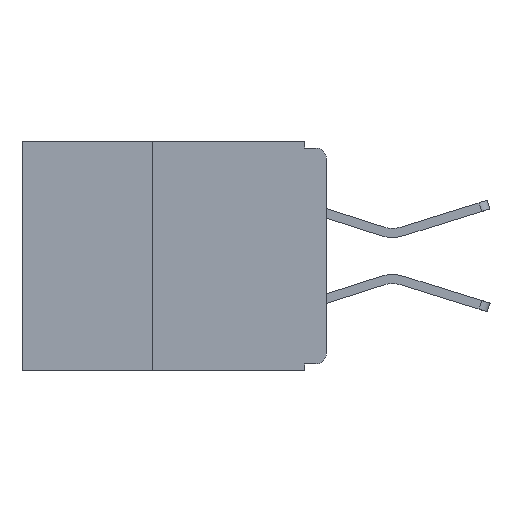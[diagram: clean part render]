
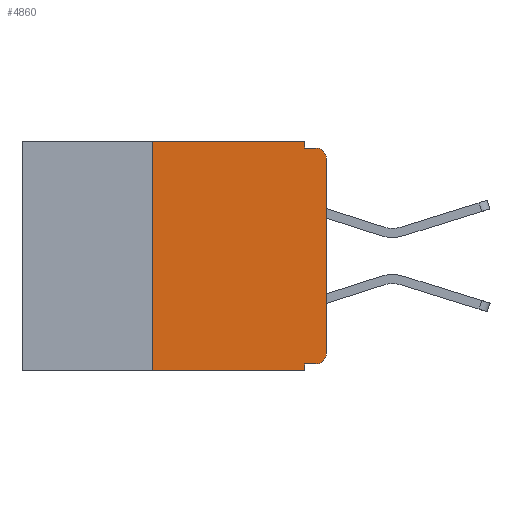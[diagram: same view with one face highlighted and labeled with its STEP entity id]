
A CAD part, left-side view. The second image highlights one B-rep face of the part: STEP entity #4860.
In plain terms, the highlighted planar face has unit normal (-1, 0, 0).
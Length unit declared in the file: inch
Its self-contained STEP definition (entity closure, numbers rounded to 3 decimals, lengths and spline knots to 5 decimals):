
#43 = LINE ( 'NONE', #23485, #11385 ) ;
#1338 = VERTEX_POINT ( 'NONE', #29481 ) ;
#1830 = LINE ( 'NONE', #26100, #28322 ) ;
#1840 = FACE_OUTER_BOUND ( 'NONE', #27056, .T. ) ;
#1933 = AXIS2_PLACEMENT_3D ( 'NONE', #18359, #2943, #20865 ) ;
#2165 = VERTEX_POINT ( 'NONE', #4716 ) ;
#2302 = VECTOR ( 'NONE', #6045, 39.37008 ) ;
#2535 = CARTESIAN_POINT ( 'NONE',  ( 0., 0.25, -0.33 ) ) ;
#2649 = CARTESIAN_POINT ( 'NONE',  ( 0., 0.25, -0.33 ) ) ;
#2943 = DIRECTION ( 'NONE',  ( -1., 0., 0. ) ) ;
#3326 = DIRECTION ( 'NONE',  ( 0., -1., 0. ) ) ;
#3347 = ORIENTED_EDGE ( 'NONE', *, *, #19460, .T. ) ;
#3734 = CARTESIAN_POINT ( 'NONE',  ( 0., 0.015, -0.025 ) ) ;
#4126 = VECTOR ( 'NONE', #15918, 39.37008 ) ;
#4716 = CARTESIAN_POINT ( 'NONE',  ( 0., 0., -0.305 ) ) ;
#4750 = CARTESIAN_POINT ( 'NONE',  ( 0., 0., -0.025 ) ) ;
#4860 = ADVANCED_FACE ( 'NONE', ( #1840 ), #25581, .F. ) ;
#4918 = EDGE_CURVE ( 'NONE', #14846, #13482, #27250, .T. ) ;
#5679 = ORIENTED_EDGE ( 'NONE', *, *, #11843, .F. ) ;
#6036 = VERTEX_POINT ( 'NONE', #6167 ) ;
#6045 = DIRECTION ( 'NONE',  ( 0., 0., -1. ) ) ;
#6167 = CARTESIAN_POINT ( 'NONE',  ( 0., 0.031, 0. ) ) ;
#6337 = DIRECTION ( 'NONE',  ( 0., 0., -1. ) ) ;
#6583 = EDGE_CURVE ( 'NONE', #7610, #16724, #1830, .T. ) ;
#6735 = ORIENTED_EDGE ( 'NONE', *, *, #13038, .F. ) ;
#7159 = VECTOR ( 'NONE', #10662, 39.37008 ) ;
#7420 = VERTEX_POINT ( 'NONE', #24932 ) ;
#7610 = VERTEX_POINT ( 'NONE', #21258 ) ;
#7653 = VECTOR ( 'NONE', #10467, 39.37008 ) ;
#9402 = CIRCLE ( 'NONE', #15820, 0.015 ) ;
#9878 = CARTESIAN_POINT ( 'NONE',  ( 0., 0.031, -0.33 ) ) ;
#10213 = LINE ( 'NONE', #18460, #4126 ) ;
#10467 = DIRECTION ( 'NONE',  ( 0., 0., 1. ) ) ;
#10662 = DIRECTION ( 'NONE',  ( 0., 1., 0. ) ) ;
#10884 = ORIENTED_EDGE ( 'NONE', *, *, #26653, .T. ) ;
#11244 = CARTESIAN_POINT ( 'NONE',  ( 0., 0.015, -0.01 ) ) ;
#11385 = VECTOR ( 'NONE', #28417, 39.37008 ) ;
#11645 = LINE ( 'NONE', #18712, #30720 ) ;
#11775 = CIRCLE ( 'NONE', #1933, 0.015 ) ;
#11843 = EDGE_CURVE ( 'NONE', #14846, #12485, #14467, .T. ) ;
#12485 = VERTEX_POINT ( 'NONE', #30921 ) ;
#13038 = EDGE_CURVE ( 'NONE', #1338, #7420, #13977, .T. ) ;
#13207 = ORIENTED_EDGE ( 'NONE', *, *, #20658, .F. ) ;
#13482 = VERTEX_POINT ( 'NONE', #9878 ) ;
#13977 = LINE ( 'NONE', #25725, #7159 ) ;
#14467 = LINE ( 'NONE', #2649, #7653 ) ;
#14846 = VERTEX_POINT ( 'NONE', #2535 ) ;
#15820 = AXIS2_PLACEMENT_3D ( 'NONE', #3734, #21602, #6337 ) ;
#15918 = DIRECTION ( 'NONE',  ( 0., 0., 1. ) ) ;
#16036 = AXIS2_PLACEMENT_3D ( 'NONE', #25434, #25361, #25319 ) ;
#16724 = VERTEX_POINT ( 'NONE', #11244 ) ;
#18359 = CARTESIAN_POINT ( 'NONE',  ( 0., 0.015, -0.305 ) ) ;
#18460 = CARTESIAN_POINT ( 'NONE',  ( 0., 0., 0. ) ) ;
#18712 = CARTESIAN_POINT ( 'NONE',  ( 0., 0.437, 0. ) ) ;
#18724 = EDGE_CURVE ( 'NONE', #6036, #7610, #43, .T. ) ;
#19101 = VERTEX_POINT ( 'NONE', #4750 ) ;
#19460 = EDGE_CURVE ( 'NONE', #19101, #16724, #9402, .T. ) ;
#20658 = EDGE_CURVE ( 'NONE', #12485, #6036, #11645, .T. ) ;
#20865 = DIRECTION ( 'NONE',  ( 0., 0., -1. ) ) ;
#21258 = CARTESIAN_POINT ( 'NONE',  ( 0., 0.031, -0.01 ) ) ;
#21354 = CARTESIAN_POINT ( 'NONE',  ( 0., 0.031, -0.33 ) ) ;
#21386 = ORIENTED_EDGE ( 'NONE', *, *, #4918, .T. ) ;
#21602 = DIRECTION ( 'NONE',  ( -1., 0., 0. ) ) ;
#23485 = CARTESIAN_POINT ( 'NONE',  ( 0., 0.031, 0. ) ) ;
#24553 = CARTESIAN_POINT ( 'NONE',  ( 0., 0.437, -0.33 ) ) ;
#24576 = DIRECTION ( 'NONE',  ( 0., -1., 0. ) ) ;
#24932 = CARTESIAN_POINT ( 'NONE',  ( 0., 0.031, -0.32 ) ) ;
#25319 = DIRECTION ( 'NONE',  ( 0., 0., -1. ) ) ;
#25361 = DIRECTION ( 'NONE',  ( 1., 0., 0. ) ) ;
#25434 = CARTESIAN_POINT ( 'NONE',  ( 0., 0.437, 0. ) ) ;
#25581 = PLANE ( 'NONE',  #16036 ) ;
#25725 = CARTESIAN_POINT ( 'NONE',  ( 0., 0., -0.32 ) ) ;
#25998 = DIRECTION ( 'NONE',  ( 0., -1., 0. ) ) ;
#26100 = CARTESIAN_POINT ( 'NONE',  ( 0., 0., -0.01 ) ) ;
#26457 = VECTOR ( 'NONE', #24576, 39.37008 ) ;
#26653 = EDGE_CURVE ( 'NONE', #1338, #2165, #11775, .T. ) ;
#26699 = EDGE_CURVE ( 'NONE', #2165, #19101, #10213, .T. ) ;
#26879 = ORIENTED_EDGE ( 'NONE', *, *, #30800, .F. ) ;
#27056 = EDGE_LOOP ( 'NONE', ( #27460, #3347, #27448, #29534, #13207, #5679, #21386, #26879, #6735, #10884 ) ) ;
#27250 = LINE ( 'NONE', #24553, #26457 ) ;
#27448 = ORIENTED_EDGE ( 'NONE', *, *, #6583, .F. ) ;
#27460 = ORIENTED_EDGE ( 'NONE', *, *, #26699, .T. ) ;
#28322 = VECTOR ( 'NONE', #25998, 39.37008 ) ;
#28416 = LINE ( 'NONE', #21354, #2302 ) ;
#28417 = DIRECTION ( 'NONE',  ( 0., 0., -1. ) ) ;
#29481 = CARTESIAN_POINT ( 'NONE',  ( 0., 0.015, -0.32 ) ) ;
#29534 = ORIENTED_EDGE ( 'NONE', *, *, #18724, .F. ) ;
#30720 = VECTOR ( 'NONE', #3326, 39.37008 ) ;
#30800 = EDGE_CURVE ( 'NONE', #7420, #13482, #28416, .T. ) ;
#30921 = CARTESIAN_POINT ( 'NONE',  ( 0., 0.25, 0. ) ) ;
